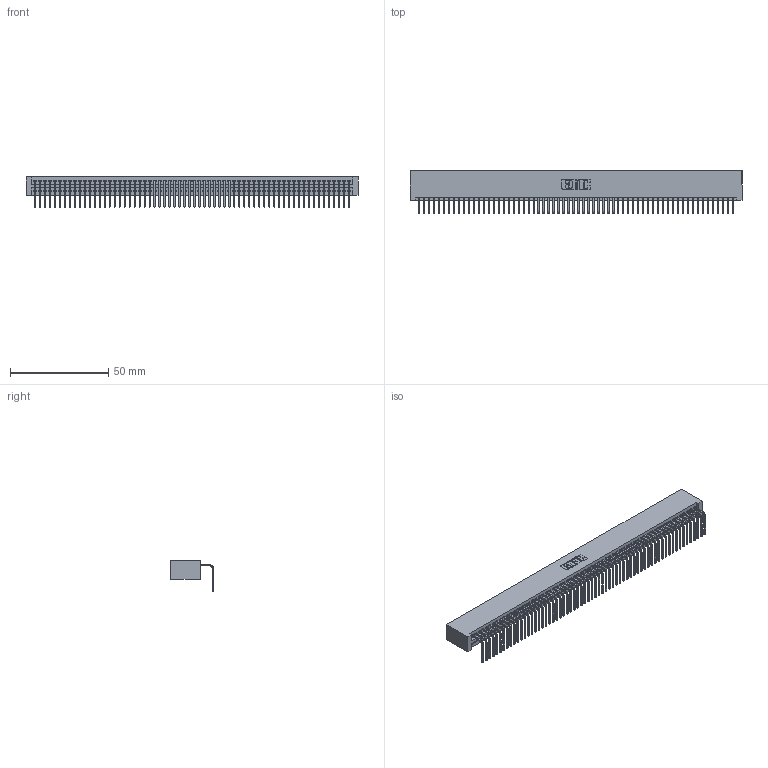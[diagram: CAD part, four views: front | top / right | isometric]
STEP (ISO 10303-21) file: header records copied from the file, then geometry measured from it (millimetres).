
FILE_DESCRIPTION (( 'STEP AP203' ), '1' );
FILE_NAME ('345-064-558-101.STEP', '2018-09-28T09:40:25', ( '' ), ( '' ), 'SwSTEP 2.0', 'SolidWorks 2016', '' );
FILE_SCHEMA (( 'CONFIG_CONTROL_DESIGN' ));
Length unit declared in the file: inch
Products named in the file (3): 345 Part_No Mounting Lugs; 345-064-558-101; 345-292-001_558 Tail - 2
Assembly tree (65 placements, depth 2):
  345-064-558-101
    345 Part_No Mounting Lugs
    345-292-001_558 Tail - 2  x64
Bounding box: 169.16 x 21.83 x 15.37 mm (x, y, z)
Volume: 17045.2 mm3; surface area: 24393.6 mm2
Topology: 65 solids, 65 shells, 3958 faces, 11965 edges, 7890 vertices
Faces by surface type: plane 2764, cylinder 1194
Entity records: 45013 total; most frequent: CARTESIAN_POINT 7804, ORIENTED_EDGE 7802, DIRECTION 6777, EDGE_CURVE 3901, LINE 3521, VECTOR 3521, VERTEX_POINT 2598, AXIS2_PLACEMENT_3D 1628
